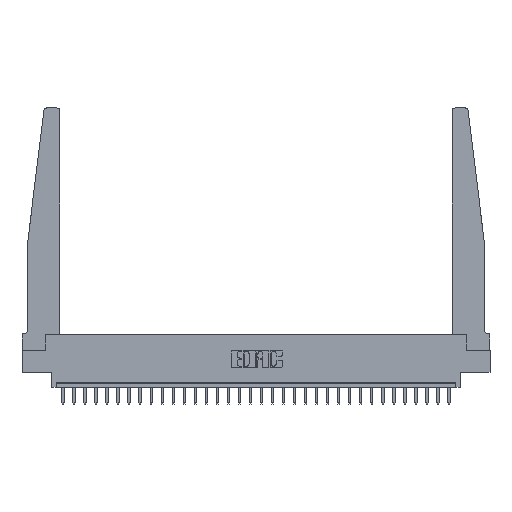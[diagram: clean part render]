
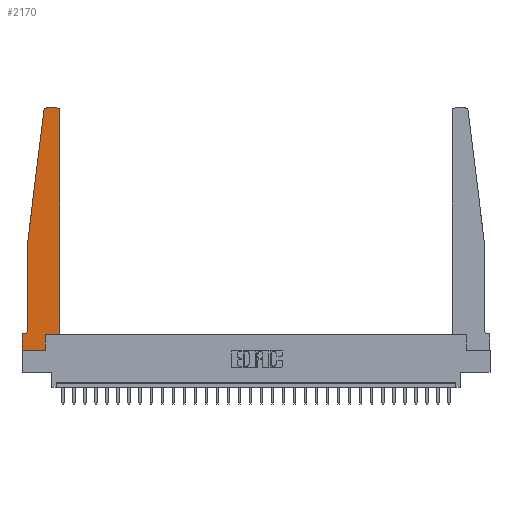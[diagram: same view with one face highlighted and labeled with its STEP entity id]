
A CAD part, top view. The second image highlights one B-rep face of the part: STEP entity #2170.
In plain terms, the highlighted planar face has unit normal (0, 0, 1).
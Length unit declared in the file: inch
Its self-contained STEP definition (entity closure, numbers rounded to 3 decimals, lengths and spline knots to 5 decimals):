
#499 = LINE ( 'NONE', #7579, #15822 ) ;
#730 = AXIS2_PLACEMENT_3D ( 'NONE', #22549, #11791, #1055 ) ;
#1055 = DIRECTION ( 'NONE',  ( 1., 0., 0. ) ) ;
#1095 = ORIENTED_EDGE ( 'NONE', *, *, #6445, .T. ) ;
#1199 = CARTESIAN_POINT ( 'NONE',  ( 0.2605, 0.18, 0.37 ) ) ;
#1427 = EDGE_CURVE ( 'NONE', #2345, #12112, #2213, .T. ) ;
#1531 = CARTESIAN_POINT ( 'NONE',  ( 0.395, 2.75, 0.37 ) ) ;
#1613 = CARTESIAN_POINT ( 'NONE',  ( 0., 0.1875, 0.37 ) ) ;
#1769 = EDGE_LOOP ( 'NONE', ( #7428, #1095, #13972, #21049, #14965, #4027, #26571, #17014, #4032, #16004, #23203, #17969 ) ) ;
#1802 = VERTEX_POINT ( 'NONE', #5704 ) ;
#2113 = DIRECTION ( 'NONE',  ( -1., 0., 0. ) ) ;
#2170 = ADVANCED_FACE ( 'NONE', ( #21946 ), #3487, .T. ) ;
#2213 = LINE ( 'NONE', #6704, #7643 ) ;
#2345 = VERTEX_POINT ( 'NONE', #17161 ) ;
#2498 = VERTEX_POINT ( 'NONE', #17732 ) ;
#2849 = LINE ( 'NONE', #18143, #24979 ) ;
#3063 = EDGE_CURVE ( 'NONE', #11272, #25063, #8230, .T. ) ;
#3387 = AXIS2_PLACEMENT_3D ( 'NONE', #19722, #8836, #13018 ) ;
#3487 = PLANE ( 'NONE',  #4050 ) ;
#3915 = VERTEX_POINT ( 'NONE', #8219 ) ;
#4027 = ORIENTED_EDGE ( 'NONE', *, *, #22838, .T. ) ;
#4032 = ORIENTED_EDGE ( 'NONE', *, *, #25370, .T. ) ;
#4050 = AXIS2_PLACEMENT_3D ( 'NONE', #1613, #10068, #16548 ) ;
#4582 = LINE ( 'NONE', #24726, #22637 ) ;
#5275 = VECTOR ( 'NONE', #23283, 39.37008 ) ;
#5401 = VERTEX_POINT ( 'NONE', #9674 ) ;
#5704 = CARTESIAN_POINT ( 'NONE',  ( 0.24675, 2.72367, 0.37 ) ) ;
#6445 = EDGE_CURVE ( 'NONE', #24930, #1802, #21441, .T. ) ;
#6566 = CARTESIAN_POINT ( 'NONE',  ( 0.065, 1.25, 0.37 ) ) ;
#6653 = DIRECTION ( 'NONE',  ( 0., 0., -1. ) ) ;
#6704 = CARTESIAN_POINT ( 'NONE',  ( 0., 0., 0.37 ) ) ;
#6853 = DIRECTION ( 'NONE',  ( 0., -1., 0. ) ) ;
#7291 = LINE ( 'NONE', #8036, #5275 ) ;
#7428 = ORIENTED_EDGE ( 'NONE', *, *, #14047, .T. ) ;
#7579 = CARTESIAN_POINT ( 'NONE',  ( 0.2605, 0.18, 0.37 ) ) ;
#7643 = VECTOR ( 'NONE', #6853, 39.37008 ) ;
#8036 = CARTESIAN_POINT ( 'NONE',  ( 0.065, 1.25, 0.37 ) ) ;
#8219 = CARTESIAN_POINT ( 'NONE',  ( 0.065, 1.25, 0.37 ) ) ;
#8230 = CIRCLE ( 'NONE', #18675, 0.05 ) ;
#8836 = DIRECTION ( 'NONE',  ( 0., 0., 1. ) ) ;
#9674 = CARTESIAN_POINT ( 'NONE',  ( 0.425, 2.72, 0.37 ) ) ;
#10068 = DIRECTION ( 'NONE',  ( 0., 0., 1. ) ) ;
#10904 = CARTESIAN_POINT ( 'NONE',  ( 0., 0., 0.37 ) ) ;
#11272 = VERTEX_POINT ( 'NONE', #18234 ) ;
#11791 = DIRECTION ( 'NONE',  ( 0., 0., 1. ) ) ;
#11824 = DIRECTION ( 'NONE',  ( -1., 0., 0. ) ) ;
#12112 = VERTEX_POINT ( 'NONE', #16560 ) ;
#12678 = DIRECTION ( 'NONE',  ( -1., 0., 0. ) ) ;
#13018 = DIRECTION ( 'NONE',  ( 1., 0., 0. ) ) ;
#13972 = ORIENTED_EDGE ( 'NONE', *, *, #24325, .T. ) ;
#14047 = EDGE_CURVE ( 'NONE', #25181, #24930, #24256, .T. ) ;
#14965 = ORIENTED_EDGE ( 'NONE', *, *, #3063, .T. ) ;
#15040 = CARTESIAN_POINT ( 'NONE',  ( 0.425, 0.18, 0.37 ) ) ;
#15653 = CARTESIAN_POINT ( 'NONE',  ( 0.2605, 0., 0.37 ) ) ;
#15822 = VECTOR ( 'NONE', #16563, 39.37008 ) ;
#16004 = ORIENTED_EDGE ( 'NONE', *, *, #24177, .T. ) ;
#16078 = VERTEX_POINT ( 'NONE', #1199 ) ;
#16548 = DIRECTION ( 'NONE',  ( 1., 0., 0. ) ) ;
#16560 = CARTESIAN_POINT ( 'NONE',  ( 0., 0., 0.37 ) ) ;
#16563 = DIRECTION ( 'NONE',  ( 0., 1., 0. ) ) ;
#17014 = ORIENTED_EDGE ( 'NONE', *, *, #24429, .T. ) ;
#17161 = CARTESIAN_POINT ( 'NONE',  ( 0., 0.1875, 0.37 ) ) ;
#17384 = DIRECTION ( 'NONE',  ( 0., -1., 0. ) ) ;
#17536 = DIRECTION ( 'NONE',  ( 0., 1., 0. ) ) ;
#17620 = CARTESIAN_POINT ( 'NONE',  ( 0.015, 0.2375, 0.37 ) ) ;
#17632 = CIRCLE ( 'NONE', #730, 0.03 ) ;
#17732 = CARTESIAN_POINT ( 'NONE',  ( 0.425, 0.18, 0.37 ) ) ;
#17969 = ORIENTED_EDGE ( 'NONE', *, *, #23473, .T. ) ;
#18143 = CARTESIAN_POINT ( 'NONE',  ( 0.065, 0.1875, 0.37 ) ) ;
#18234 = CARTESIAN_POINT ( 'NONE',  ( 0.065, 0.2375, 0.37 ) ) ;
#18675 = AXIS2_PLACEMENT_3D ( 'NONE', #17620, #6653, #12678 ) ;
#19569 = CARTESIAN_POINT ( 'NONE',  ( 0.25, 2.75, 0.37 ) ) ;
#19722 = CARTESIAN_POINT ( 'NONE',  ( 0.27653, 2.72, 0.37 ) ) ;
#20645 = VECTOR ( 'NONE', #17536, 39.37008 ) ;
#21049 = ORIENTED_EDGE ( 'NONE', *, *, #21512, .T. ) ;
#21116 = VERTEX_POINT ( 'NONE', #15653 ) ;
#21441 = CIRCLE ( 'NONE', #3387, 0.03 ) ;
#21512 = EDGE_CURVE ( 'NONE', #3915, #11272, #22998, .T. ) ;
#21863 = DIRECTION ( 'NONE',  ( 1., 0., 0. ) ) ;
#21946 = FACE_OUTER_BOUND ( 'NONE', #1769, .T. ) ;
#22549 = CARTESIAN_POINT ( 'NONE',  ( 0.395, 2.72, 0.37 ) ) ;
#22626 = DIRECTION ( 'NONE',  ( 1., 0., 0. ) ) ;
#22637 = VECTOR ( 'NONE', #22626, 39.37008 ) ;
#22670 = VECTOR ( 'NONE', #17384, 39.37008 ) ;
#22838 = EDGE_CURVE ( 'NONE', #25063, #2345, #2849, .T. ) ;
#22998 = LINE ( 'NONE', #6566, #22670 ) ;
#23203 = ORIENTED_EDGE ( 'NONE', *, *, #23810, .T. ) ;
#23283 = DIRECTION ( 'NONE',  ( -0.122, -0.992, 0. ) ) ;
#23473 = EDGE_CURVE ( 'NONE', #5401, #25181, #17632, .T. ) ;
#23810 = EDGE_CURVE ( 'NONE', #2498, #5401, #25701, .T. ) ;
#24177 = EDGE_CURVE ( 'NONE', #16078, #2498, #4582, .T. ) ;
#24256 = LINE ( 'NONE', #19569, #27645 ) ;
#24320 = VECTOR ( 'NONE', #21863, 39.37008 ) ;
#24325 = EDGE_CURVE ( 'NONE', #1802, #3915, #7291, .T. ) ;
#24429 = EDGE_CURVE ( 'NONE', #12112, #21116, #27753, .T. ) ;
#24726 = CARTESIAN_POINT ( 'NONE',  ( 0.425, 0.18, 0.37 ) ) ;
#24930 = VERTEX_POINT ( 'NONE', #27593 ) ;
#24979 = VECTOR ( 'NONE', #11824, 39.37008 ) ;
#25063 = VERTEX_POINT ( 'NONE', #25696 ) ;
#25181 = VERTEX_POINT ( 'NONE', #1531 ) ;
#25370 = EDGE_CURVE ( 'NONE', #21116, #16078, #499, .T. ) ;
#25696 = CARTESIAN_POINT ( 'NONE',  ( 0.015, 0.1875, 0.37 ) ) ;
#25701 = LINE ( 'NONE', #15040, #20645 ) ;
#26571 = ORIENTED_EDGE ( 'NONE', *, *, #1427, .T. ) ;
#27593 = CARTESIAN_POINT ( 'NONE',  ( 0.27653, 2.75, 0.37 ) ) ;
#27645 = VECTOR ( 'NONE', #2113, 39.37008 ) ;
#27753 = LINE ( 'NONE', #10904, #24320 ) ;
